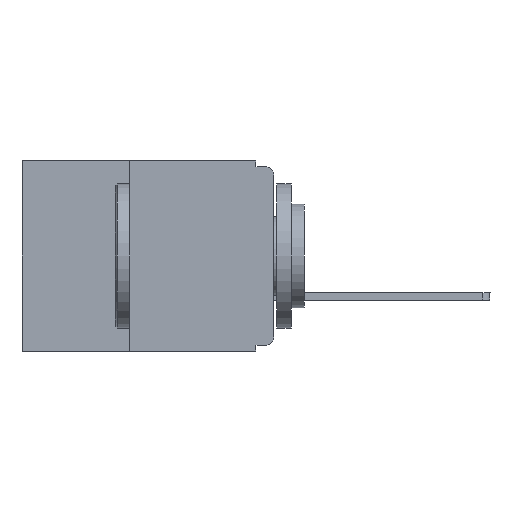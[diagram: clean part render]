
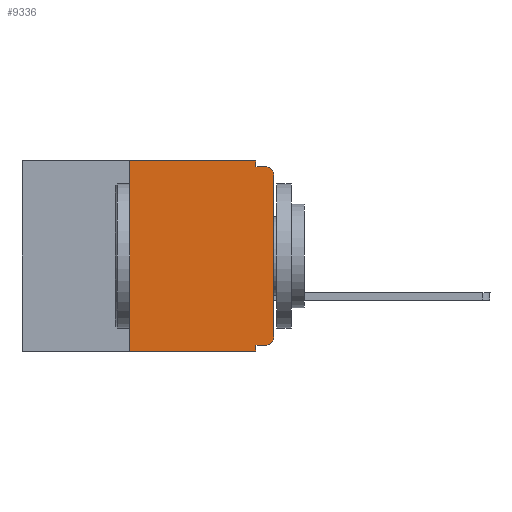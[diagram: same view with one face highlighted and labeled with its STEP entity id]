
A CAD part, left-side view. The second image highlights one B-rep face of the part: STEP entity #9336.
In plain terms, the highlighted planar face has unit normal (-1, 0, 0).
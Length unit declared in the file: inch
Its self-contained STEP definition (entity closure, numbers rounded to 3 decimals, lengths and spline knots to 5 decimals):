
#31 = CARTESIAN_POINT ( 'NONE',  ( 0., 0.015, -0.305 ) ) ;
#310 = DIRECTION ( 'NONE',  ( 1., 0., 0. ) ) ;
#583 = CARTESIAN_POINT ( 'NONE',  ( 0., 0.031, 0. ) ) ;
#664 = LINE ( 'NONE', #10554, #14981 ) ;
#917 = VECTOR ( 'NONE', #13317, 39.37008 ) ;
#1078 = VERTEX_POINT ( 'NONE', #9853 ) ;
#1225 = LINE ( 'NONE', #6978, #14079 ) ;
#1360 = DIRECTION ( 'NONE',  ( -1., 0., 0. ) ) ;
#1508 = CARTESIAN_POINT ( 'NONE',  ( 0., 0.25, 0. ) ) ;
#1684 = LINE ( 'NONE', #14234, #5113 ) ;
#1705 = DIRECTION ( 'NONE',  ( 0., 0., -1. ) ) ;
#1778 = EDGE_CURVE ( 'NONE', #1078, #10823, #2360, .T. ) ;
#2118 = AXIS2_PLACEMENT_3D ( 'NONE', #2742, #8459, #1705 ) ;
#2208 = CARTESIAN_POINT ( 'NONE',  ( 0., 0.031, -0.33 ) ) ;
#2301 = DIRECTION ( 'NONE',  ( 0., 0., -1. ) ) ;
#2360 = LINE ( 'NONE', #6829, #10824 ) ;
#2531 = AXIS2_PLACEMENT_3D ( 'NONE', #10344, #310, #2301 ) ;
#2720 = EDGE_CURVE ( 'NONE', #8908, #7669, #5005, .T. ) ;
#2742 = CARTESIAN_POINT ( 'NONE',  ( 0., 0.015, -0.025 ) ) ;
#2915 = LINE ( 'NONE', #583, #917 ) ;
#3052 = EDGE_CURVE ( 'NONE', #4162, #9455, #664, .T. ) ;
#3095 = EDGE_CURVE ( 'NONE', #8504, #6367, #1225, .T. ) ;
#3169 = CIRCLE ( 'NONE', #6583, 0.015 ) ;
#3288 = ORIENTED_EDGE ( 'NONE', *, *, #3095, .F. ) ;
#3684 = DIRECTION ( 'NONE',  ( 0., 1., 0. ) ) ;
#3693 = CARTESIAN_POINT ( 'NONE',  ( 0., 0.015, -0.01 ) ) ;
#4162 = VERTEX_POINT ( 'NONE', #11515 ) ;
#4226 = CARTESIAN_POINT ( 'NONE',  ( 0., 0.031, 0. ) ) ;
#4475 = VECTOR ( 'NONE', #10952, 39.37008 ) ;
#4588 = VECTOR ( 'NONE', #12651, 39.37008 ) ;
#4750 = ORIENTED_EDGE ( 'NONE', *, *, #14953, .F. ) ;
#4791 = EDGE_CURVE ( 'NONE', #1078, #6530, #3169, .T. ) ;
#4941 = LINE ( 'NONE', #6922, #4588 ) ;
#5005 = LINE ( 'NONE', #7462, #4475 ) ;
#5113 = VECTOR ( 'NONE', #7420, 39.37008 ) ;
#5637 = VECTOR ( 'NONE', #12483, 39.37008 ) ;
#6367 = VERTEX_POINT ( 'NONE', #3693 ) ;
#6530 = VERTEX_POINT ( 'NONE', #13811 ) ;
#6583 = AXIS2_PLACEMENT_3D ( 'NONE', #31, #1360, #10791 ) ;
#6829 = CARTESIAN_POINT ( 'NONE',  ( 0., 0., -0.32 ) ) ;
#6838 = ORIENTED_EDGE ( 'NONE', *, *, #1778, .F. ) ;
#6922 = CARTESIAN_POINT ( 'NONE',  ( 0., 0., 0. ) ) ;
#6978 = CARTESIAN_POINT ( 'NONE',  ( 0., 0., -0.01 ) ) ;
#7090 = ORIENTED_EDGE ( 'NONE', *, *, #2720, .F. ) ;
#7252 = ORIENTED_EDGE ( 'NONE', *, *, #7510, .T. ) ;
#7386 = CIRCLE ( 'NONE', #2118, 0.015 ) ;
#7420 = DIRECTION ( 'NONE',  ( 0., 0., 1. ) ) ;
#7462 = CARTESIAN_POINT ( 'NONE',  ( 0., 0.437, 0. ) ) ;
#7510 = EDGE_CURVE ( 'NONE', #14821, #6367, #7386, .T. ) ;
#7669 = VERTEX_POINT ( 'NONE', #4226 ) ;
#7881 = ORIENTED_EDGE ( 'NONE', *, *, #4791, .T. ) ;
#7938 = ORIENTED_EDGE ( 'NONE', *, *, #11227, .F. ) ;
#8452 = CARTESIAN_POINT ( 'NONE',  ( 0., 0.031, -0.32 ) ) ;
#8459 = DIRECTION ( 'NONE',  ( -1., 0., 0. ) ) ;
#8504 = VERTEX_POINT ( 'NONE', #13785 ) ;
#8908 = VERTEX_POINT ( 'NONE', #1508 ) ;
#8947 = ORIENTED_EDGE ( 'NONE', *, *, #10944, .T. ) ;
#9336 = ADVANCED_FACE ( 'NONE', ( #9719 ), #12563, .F. ) ;
#9455 = VERTEX_POINT ( 'NONE', #11084 ) ;
#9719 = FACE_OUTER_BOUND ( 'NONE', #12574, .T. ) ;
#9853 = CARTESIAN_POINT ( 'NONE',  ( 0., 0.015, -0.32 ) ) ;
#10344 = CARTESIAN_POINT ( 'NONE',  ( 0., 0.437, 0. ) ) ;
#10554 = CARTESIAN_POINT ( 'NONE',  ( 0., 0.437, -0.33 ) ) ;
#10791 = DIRECTION ( 'NONE',  ( 0., 0., -1. ) ) ;
#10823 = VERTEX_POINT ( 'NONE', #8452 ) ;
#10824 = VECTOR ( 'NONE', #3684, 39.37008 ) ;
#10870 = ORIENTED_EDGE ( 'NONE', *, *, #14016, .F. ) ;
#10944 = EDGE_CURVE ( 'NONE', #6530, #14821, #4941, .T. ) ;
#10952 = DIRECTION ( 'NONE',  ( 0., -1., 0. ) ) ;
#11084 = CARTESIAN_POINT ( 'NONE',  ( 0., 0.031, -0.33 ) ) ;
#11227 = EDGE_CURVE ( 'NONE', #4162, #8908, #1684, .T. ) ;
#11515 = CARTESIAN_POINT ( 'NONE',  ( 0., 0.25, -0.33 ) ) ;
#11807 = ORIENTED_EDGE ( 'NONE', *, *, #3052, .T. ) ;
#11965 = LINE ( 'NONE', #2208, #5637 ) ;
#12483 = DIRECTION ( 'NONE',  ( 0., 0., -1. ) ) ;
#12563 = PLANE ( 'NONE',  #2531 ) ;
#12574 = EDGE_LOOP ( 'NONE', ( #8947, #7252, #3288, #4750, #7090, #7938, #11807, #10870, #6838, #7881 ) ) ;
#12651 = DIRECTION ( 'NONE',  ( 0., 0., 1. ) ) ;
#12856 = DIRECTION ( 'NONE',  ( 0., -1., 0. ) ) ;
#13161 = DIRECTION ( 'NONE',  ( 0., -1., 0. ) ) ;
#13317 = DIRECTION ( 'NONE',  ( 0., 0., -1. ) ) ;
#13785 = CARTESIAN_POINT ( 'NONE',  ( 0., 0.031, -0.01 ) ) ;
#13811 = CARTESIAN_POINT ( 'NONE',  ( 0., 0., -0.305 ) ) ;
#14012 = CARTESIAN_POINT ( 'NONE',  ( 0., 0., -0.025 ) ) ;
#14016 = EDGE_CURVE ( 'NONE', #10823, #9455, #11965, .T. ) ;
#14079 = VECTOR ( 'NONE', #13161, 39.37008 ) ;
#14234 = CARTESIAN_POINT ( 'NONE',  ( 0., 0.25, -0.33 ) ) ;
#14821 = VERTEX_POINT ( 'NONE', #14012 ) ;
#14953 = EDGE_CURVE ( 'NONE', #7669, #8504, #2915, .T. ) ;
#14981 = VECTOR ( 'NONE', #12856, 39.37008 ) ;
